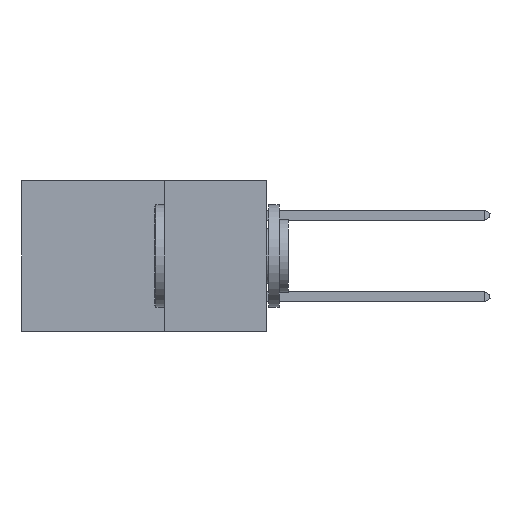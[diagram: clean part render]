
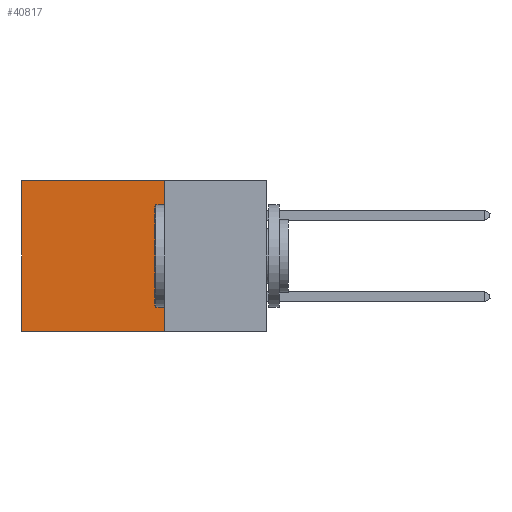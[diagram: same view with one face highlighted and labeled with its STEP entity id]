
A CAD part, left-side view. The second image highlights one B-rep face of the part: STEP entity #40817.
In plain terms, the highlighted planar face has unit normal (-1, 0, 0).
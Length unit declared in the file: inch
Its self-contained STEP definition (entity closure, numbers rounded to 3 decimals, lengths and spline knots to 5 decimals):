
#1056 = EDGE_LOOP ( 'NONE', ( #27745, #43680, #12502, #18340 ) ) ;
#2829 = LINE ( 'NONE', #19660, #21444 ) ;
#6985 = EDGE_CURVE ( 'NONE', #30892, #36785, #2829, .T. ) ;
#7070 = VERTEX_POINT ( 'NONE', #30946 ) ;
#7524 = VECTOR ( 'NONE', #43077, 39.37008 ) ;
#8275 = VECTOR ( 'NONE', #23905, 39.37008 ) ;
#9756 = CARTESIAN_POINT ( 'NONE',  ( 0.2875, 0.25, 0. ) ) ;
#12502 = ORIENTED_EDGE ( 'NONE', *, *, #21513, .F. ) ;
#12766 = DIRECTION ( 'NONE',  ( 0., 0., -1. ) ) ;
#13049 = VECTOR ( 'NONE', #12766, 39.37008 ) ;
#13382 = LINE ( 'NONE', #39373, #7524 ) ;
#15933 = DIRECTION ( 'NONE',  ( 0., 1., 0. ) ) ;
#16353 = EDGE_CURVE ( 'NONE', #7070, #36785, #41357, .T. ) ;
#16722 = PLANE ( 'NONE',  #43113 ) ;
#17177 = VERTEX_POINT ( 'NONE', #9756 ) ;
#17981 = EDGE_CURVE ( 'NONE', #17177, #7070, #18175, .T. ) ;
#18175 = LINE ( 'NONE', #20205, #8275 ) ;
#18340 = ORIENTED_EDGE ( 'NONE', *, *, #17981, .T. ) ;
#19660 = CARTESIAN_POINT ( 'NONE',  ( 0.2875, 0.25, -0.37 ) ) ;
#20205 = CARTESIAN_POINT ( 'NONE',  ( 0.2875, 0.25, 0. ) ) ;
#20451 = CARTESIAN_POINT ( 'NONE',  ( 0.2875, 0.25, 0. ) ) ;
#21444 = VECTOR ( 'NONE', #15933, 39.37008 ) ;
#21513 = EDGE_CURVE ( 'NONE', #17177, #30892, #13382, .T. ) ;
#23905 = DIRECTION ( 'NONE',  ( 0., 1., 0. ) ) ;
#24144 = DIRECTION ( 'NONE',  ( 0., 0., -1. ) ) ;
#24907 = CARTESIAN_POINT ( 'NONE',  ( 0.2875, 0.25, -0.37 ) ) ;
#27745 = ORIENTED_EDGE ( 'NONE', *, *, #16353, .T. ) ;
#30892 = VERTEX_POINT ( 'NONE', #24907 ) ;
#30946 = CARTESIAN_POINT ( 'NONE',  ( 0.2875, 0.6, 0. ) ) ;
#33639 = CARTESIAN_POINT ( 'NONE',  ( 0.2875, 0.6, -0.37 ) ) ;
#36230 = FACE_OUTER_BOUND ( 'NONE', #1056, .T. ) ;
#36785 = VERTEX_POINT ( 'NONE', #33639 ) ;
#38598 = CARTESIAN_POINT ( 'NONE',  ( 0.2875, 0.6, 0. ) ) ;
#39373 = CARTESIAN_POINT ( 'NONE',  ( 0.2875, 0.25, 0. ) ) ;
#40817 = ADVANCED_FACE ( 'NONE', ( #36230 ), #16722, .F. ) ;
#41357 = LINE ( 'NONE', #38598, #13049 ) ;
#43077 = DIRECTION ( 'NONE',  ( 0., 0., -1. ) ) ;
#43113 = AXIS2_PLACEMENT_3D ( 'NONE', #20451, #46220, #24144 ) ;
#43680 = ORIENTED_EDGE ( 'NONE', *, *, #6985, .F. ) ;
#46220 = DIRECTION ( 'NONE',  ( 1., 0., 0. ) ) ;
